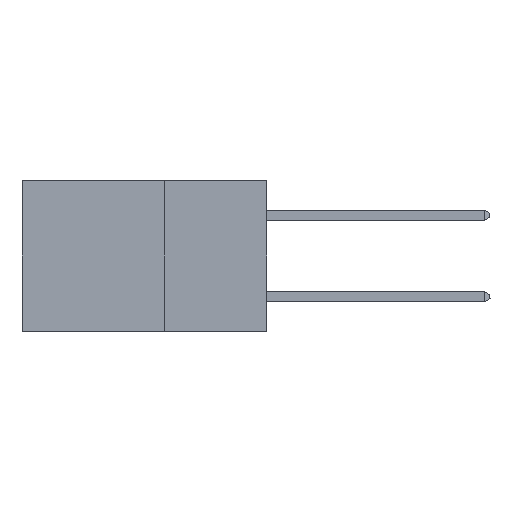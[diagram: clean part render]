
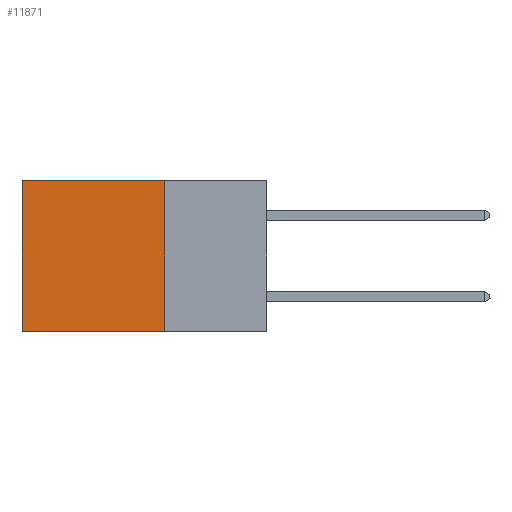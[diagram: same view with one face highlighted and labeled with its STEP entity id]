
A CAD part, left-side view. The second image highlights one B-rep face of the part: STEP entity #11871.
In plain terms, the highlighted planar face has unit normal (-1, 0, 0).
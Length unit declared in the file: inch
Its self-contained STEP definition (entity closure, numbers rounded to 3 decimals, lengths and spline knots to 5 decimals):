
#490 = DIRECTION ( 'NONE',  ( 0., 1., 0. ) ) ;
#664 = EDGE_CURVE ( 'NONE', #5432, #11038, #9695, .T. ) ;
#1196 = DIRECTION ( 'NONE',  ( 0., 0., -1. ) ) ;
#1412 = CARTESIAN_POINT ( 'NONE',  ( 0.2875, 0.25, 0. ) ) ;
#1632 = LINE ( 'NONE', #4957, #12902 ) ;
#2256 = CARTESIAN_POINT ( 'NONE',  ( 0.2875, 0.6, 0. ) ) ;
#2827 = CARTESIAN_POINT ( 'NONE',  ( 0.2875, 0.6, 0. ) ) ;
#2862 = VERTEX_POINT ( 'NONE', #5678 ) ;
#3170 = EDGE_CURVE ( 'NONE', #5432, #3364, #1632, .T. ) ;
#3223 = CARTESIAN_POINT ( 'NONE',  ( 0.2875, 0.25, -0.37 ) ) ;
#3364 = VERTEX_POINT ( 'NONE', #3223 ) ;
#3558 = DIRECTION ( 'NONE',  ( 0., 0., -1. ) ) ;
#3610 = LINE ( 'NONE', #7349, #9875 ) ;
#4235 = CARTESIAN_POINT ( 'NONE',  ( 0.2875, 0.25, 0. ) ) ;
#4957 = CARTESIAN_POINT ( 'NONE',  ( 0.2875, 0.25, 0. ) ) ;
#5068 = EDGE_CURVE ( 'NONE', #11038, #2862, #9234, .T. ) ;
#5384 = DIRECTION ( 'NONE',  ( 0., 0., -1. ) ) ;
#5432 = VERTEX_POINT ( 'NONE', #1412 ) ;
#5549 = EDGE_CURVE ( 'NONE', #3364, #2862, #3610, .T. ) ;
#5678 = CARTESIAN_POINT ( 'NONE',  ( 0.2875, 0.6, -0.37 ) ) ;
#6874 = VECTOR ( 'NONE', #10381, 39.37008 ) ;
#7349 = CARTESIAN_POINT ( 'NONE',  ( 0.2875, 0.25, -0.37 ) ) ;
#8047 = ORIENTED_EDGE ( 'NONE', *, *, #5068, .T. ) ;
#8163 = ORIENTED_EDGE ( 'NONE', *, *, #5549, .F. ) ;
#8172 = ORIENTED_EDGE ( 'NONE', *, *, #3170, .F. ) ;
#8179 = ORIENTED_EDGE ( 'NONE', *, *, #664, .T. ) ;
#8413 = FACE_OUTER_BOUND ( 'NONE', #13425, .T. ) ;
#9234 = LINE ( 'NONE', #2827, #12016 ) ;
#9695 = LINE ( 'NONE', #11896, #6874 ) ;
#9875 = VECTOR ( 'NONE', #490, 39.37008 ) ;
#10381 = DIRECTION ( 'NONE',  ( 0., 1., 0. ) ) ;
#10495 = AXIS2_PLACEMENT_3D ( 'NONE', #4235, #11884, #5384 ) ;
#10834 = PLANE ( 'NONE',  #10495 ) ;
#11038 = VERTEX_POINT ( 'NONE', #2256 ) ;
#11871 = ADVANCED_FACE ( 'NONE', ( #8413 ), #10834, .F. ) ;
#11884 = DIRECTION ( 'NONE',  ( 1., 0., 0. ) ) ;
#11896 = CARTESIAN_POINT ( 'NONE',  ( 0.2875, 0.25, 0. ) ) ;
#12016 = VECTOR ( 'NONE', #1196, 39.37008 ) ;
#12902 = VECTOR ( 'NONE', #3558, 39.37008 ) ;
#13425 = EDGE_LOOP ( 'NONE', ( #8047, #8163, #8172, #8179 ) ) ;
